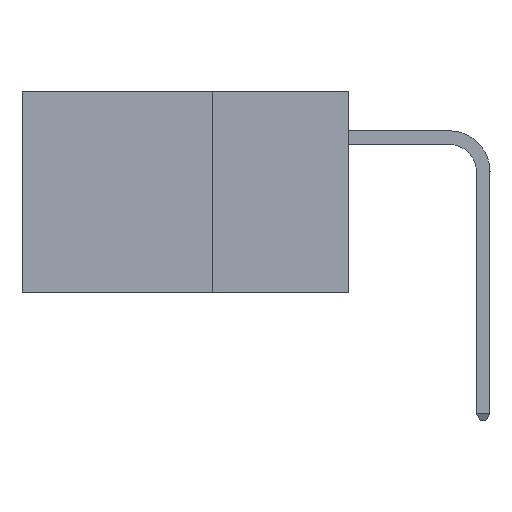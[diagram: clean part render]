
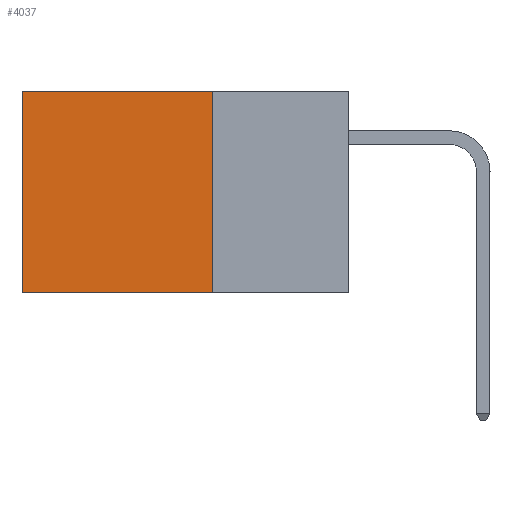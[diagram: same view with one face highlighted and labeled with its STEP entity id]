
A CAD part, left-side view. The second image highlights one B-rep face of the part: STEP entity #4037.
In plain terms, the highlighted planar face has unit normal (-1, 0, 0).
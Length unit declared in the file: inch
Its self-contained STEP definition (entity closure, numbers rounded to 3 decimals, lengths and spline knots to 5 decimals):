
#1748 = VECTOR ( 'NONE', #8013, 39.37008 ) ;
#2220 = CARTESIAN_POINT ( 'NONE',  ( 0.2875, 0.25, 0. ) ) ;
#4037 = ADVANCED_FACE ( 'NONE', ( #26882 ), #30366, .F. ) ;
#4226 = EDGE_LOOP ( 'NONE', ( #26113, #15570, #9027, #6064 ) ) ;
#5363 = AXIS2_PLACEMENT_3D ( 'NONE', #31983, #29710, #29612 ) ;
#5402 = VECTOR ( 'NONE', #27344, 39.37008 ) ;
#6064 = ORIENTED_EDGE ( 'NONE', *, *, #21735, .T. ) ;
#6476 = CARTESIAN_POINT ( 'NONE',  ( 0.2875, 0.6, 0. ) ) ;
#8013 = DIRECTION ( 'NONE',  ( 0., 0., -1. ) ) ;
#8211 = DIRECTION ( 'NONE',  ( 0., 1., 0. ) ) ;
#8439 = VERTEX_POINT ( 'NONE', #9366 ) ;
#8614 = CARTESIAN_POINT ( 'NONE',  ( 0.2875, 0.25, -0.37 ) ) ;
#9027 = ORIENTED_EDGE ( 'NONE', *, *, #28732, .F. ) ;
#9366 = CARTESIAN_POINT ( 'NONE',  ( 0.2875, 0.6, -0.37 ) ) ;
#9434 = EDGE_CURVE ( 'NONE', #10380, #8439, #13145, .T. ) ;
#10380 = VERTEX_POINT ( 'NONE', #22585 ) ;
#11664 = VERTEX_POINT ( 'NONE', #14962 ) ;
#12308 = LINE ( 'NONE', #2220, #5402 ) ;
#13145 = LINE ( 'NONE', #8614, #13979 ) ;
#13200 = CARTESIAN_POINT ( 'NONE',  ( 0.2875, 0.25, 0. ) ) ;
#13979 = VECTOR ( 'NONE', #8211, 39.37008 ) ;
#14962 = CARTESIAN_POINT ( 'NONE',  ( 0.2875, 0.25, 0. ) ) ;
#15570 = ORIENTED_EDGE ( 'NONE', *, *, #9434, .F. ) ;
#16100 = EDGE_CURVE ( 'NONE', #26684, #8439, #16145, .T. ) ;
#16145 = LINE ( 'NONE', #17825, #28337 ) ;
#17825 = CARTESIAN_POINT ( 'NONE',  ( 0.2875, 0.6, 0. ) ) ;
#18385 = DIRECTION ( 'NONE',  ( 0., 0., -1. ) ) ;
#21735 = EDGE_CURVE ( 'NONE', #11664, #26684, #12308, .T. ) ;
#22585 = CARTESIAN_POINT ( 'NONE',  ( 0.2875, 0.25, -0.37 ) ) ;
#22748 = LINE ( 'NONE', #13200, #1748 ) ;
#26113 = ORIENTED_EDGE ( 'NONE', *, *, #16100, .T. ) ;
#26684 = VERTEX_POINT ( 'NONE', #6476 ) ;
#26882 = FACE_OUTER_BOUND ( 'NONE', #4226, .T. ) ;
#27344 = DIRECTION ( 'NONE',  ( 0., 1., 0. ) ) ;
#28337 = VECTOR ( 'NONE', #18385, 39.37008 ) ;
#28732 = EDGE_CURVE ( 'NONE', #11664, #10380, #22748, .T. ) ;
#29612 = DIRECTION ( 'NONE',  ( 0., 0., -1. ) ) ;
#29710 = DIRECTION ( 'NONE',  ( 1., 0., 0. ) ) ;
#30366 = PLANE ( 'NONE',  #5363 ) ;
#31983 = CARTESIAN_POINT ( 'NONE',  ( 0.2875, 0.25, 0. ) ) ;
